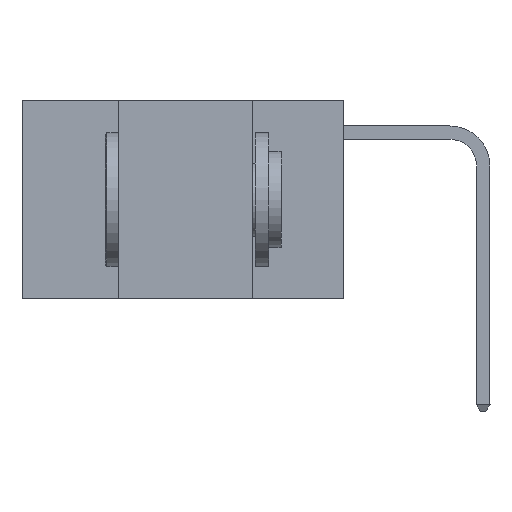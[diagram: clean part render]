
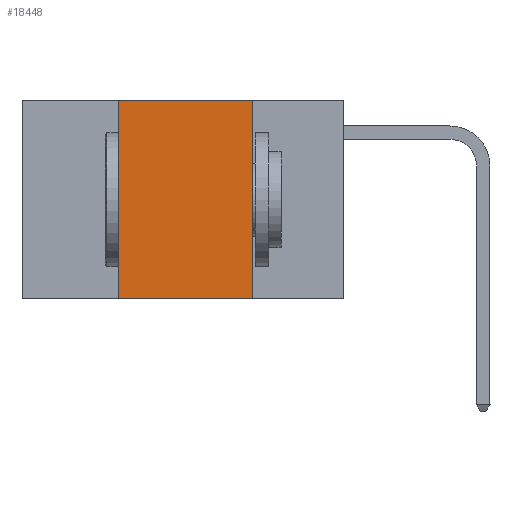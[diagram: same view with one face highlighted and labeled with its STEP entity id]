
A CAD part, left-side view. The second image highlights one B-rep face of the part: STEP entity #18448.
In plain terms, the highlighted planar face has unit normal (-1, 0, 0).
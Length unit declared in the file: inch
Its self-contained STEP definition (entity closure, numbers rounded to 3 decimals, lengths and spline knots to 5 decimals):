
#390 = ORIENTED_EDGE ( 'NONE', *, *, #30079, .F. ) ;
#827 = DIRECTION ( 'NONE',  ( 0., 0., -1. ) ) ;
#1429 = DIRECTION ( 'NONE',  ( 0., -1., 0. ) ) ;
#1660 = CARTESIAN_POINT ( 'NONE',  ( 0., 0.6, 0. ) ) ;
#2642 = EDGE_LOOP ( 'NONE', ( #23526, #5264, #390, #6775 ) ) ;
#3335 = CARTESIAN_POINT ( 'NONE',  ( 0., 0.17, 0. ) ) ;
#4913 = PLANE ( 'NONE',  #22732 ) ;
#5264 = ORIENTED_EDGE ( 'NONE', *, *, #11523, .F. ) ;
#5611 = EDGE_CURVE ( 'NONE', #13578, #9070, #14563, .T. ) ;
#6775 = ORIENTED_EDGE ( 'NONE', *, *, #22193, .T. ) ;
#7376 = VERTEX_POINT ( 'NONE', #14442 ) ;
#8691 = DIRECTION ( 'NONE',  ( 0., 0., 1. ) ) ;
#9070 = VERTEX_POINT ( 'NONE', #9173 ) ;
#9173 = CARTESIAN_POINT ( 'NONE',  ( 0., 0.17, -0.37 ) ) ;
#11523 = EDGE_CURVE ( 'NONE', #7376, #13578, #17996, .T. ) ;
#13578 = VERTEX_POINT ( 'NONE', #3335 ) ;
#14442 = CARTESIAN_POINT ( 'NONE',  ( 0., 0.42, 0. ) ) ;
#14505 = DIRECTION ( 'NONE',  ( 0., 0., -1. ) ) ;
#14546 = CARTESIAN_POINT ( 'NONE',  ( 0., 0.42, -0.37 ) ) ;
#14563 = LINE ( 'NONE', #15130, #26456 ) ;
#15130 = CARTESIAN_POINT ( 'NONE',  ( 0., 0.17, 0. ) ) ;
#15355 = LINE ( 'NONE', #27684, #21716 ) ;
#15726 = CARTESIAN_POINT ( 'NONE',  ( 0., 0.6, -0.37 ) ) ;
#17996 = LINE ( 'NONE', #1660, #23583 ) ;
#18448 = ADVANCED_FACE ( 'NONE', ( #21371 ), #4913, .F. ) ;
#21371 = FACE_OUTER_BOUND ( 'NONE', #2642, .T. ) ;
#21716 = VECTOR ( 'NONE', #8691, 39.37008 ) ;
#21904 = VECTOR ( 'NONE', #1429, 39.37008 ) ;
#22193 = EDGE_CURVE ( 'NONE', #29050, #9070, #22633, .T. ) ;
#22633 = LINE ( 'NONE', #15726, #21904 ) ;
#22732 = AXIS2_PLACEMENT_3D ( 'NONE', #26353, #28708, #14505 ) ;
#23526 = ORIENTED_EDGE ( 'NONE', *, *, #5611, .F. ) ;
#23583 = VECTOR ( 'NONE', #30125, 39.37008 ) ;
#26353 = CARTESIAN_POINT ( 'NONE',  ( 0., 0.6, 0. ) ) ;
#26456 = VECTOR ( 'NONE', #827, 39.37008 ) ;
#27684 = CARTESIAN_POINT ( 'NONE',  ( 0., 0.42, 0. ) ) ;
#28708 = DIRECTION ( 'NONE',  ( 1., 0., 0. ) ) ;
#29050 = VERTEX_POINT ( 'NONE', #14546 ) ;
#30079 = EDGE_CURVE ( 'NONE', #29050, #7376, #15355, .T. ) ;
#30125 = DIRECTION ( 'NONE',  ( 0., -1., 0. ) ) ;
